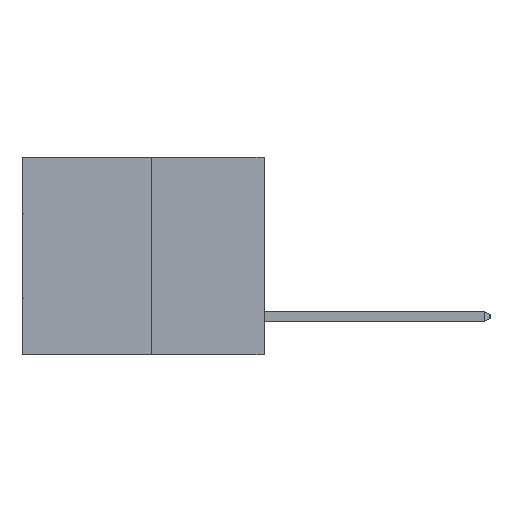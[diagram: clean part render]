
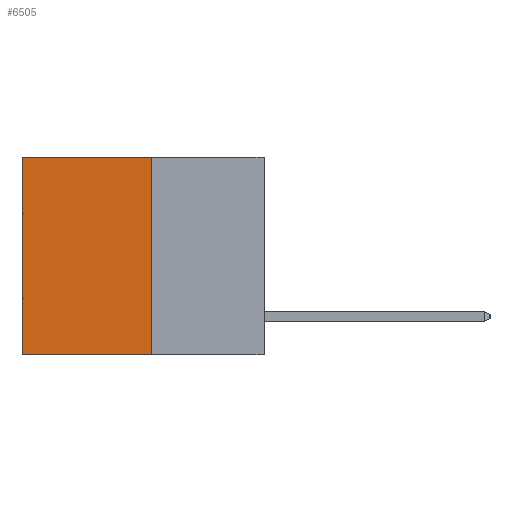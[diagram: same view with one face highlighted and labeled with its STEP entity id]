
A CAD part, left-side view. The second image highlights one B-rep face of the part: STEP entity #6505.
In plain terms, the highlighted planar face has unit normal (-1, 0, 0).
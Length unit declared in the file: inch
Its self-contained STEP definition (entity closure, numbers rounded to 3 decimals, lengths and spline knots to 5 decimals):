
#499 = FACE_OUTER_BOUND ( 'NONE', #31432, .T. ) ;
#2047 = EDGE_CURVE ( 'NONE', #15232, #29838, #20051, .T. ) ;
#3151 = LINE ( 'NONE', #14437, #3948 ) ;
#3948 = VECTOR ( 'NONE', #19595, 39.37008 ) ;
#3957 = VECTOR ( 'NONE', #15817, 39.37008 ) ;
#4215 = CARTESIAN_POINT ( 'NONE',  ( 0.3165, 0.6, 0. ) ) ;
#4527 = DIRECTION ( 'NONE',  ( 0., 0., -1. ) ) ;
#4625 = CARTESIAN_POINT ( 'NONE',  ( 0.3165, 0.28, 0. ) ) ;
#6505 = ADVANCED_FACE ( 'NONE', ( #499 ), #17336, .F. ) ;
#6701 = ORIENTED_EDGE ( 'NONE', *, *, #32404, .T. ) ;
#11124 = CARTESIAN_POINT ( 'NONE',  ( 0.3165, 0.6, -0.49 ) ) ;
#12651 = VERTEX_POINT ( 'NONE', #23319 ) ;
#14437 = CARTESIAN_POINT ( 'NONE',  ( 0.3165, 0.28, -0.49 ) ) ;
#15173 = EDGE_CURVE ( 'NONE', #12651, #21484, #23212, .T. ) ;
#15232 = VERTEX_POINT ( 'NONE', #22230 ) ;
#15817 = DIRECTION ( 'NONE',  ( 0., 0., -1. ) ) ;
#16692 = CARTESIAN_POINT ( 'NONE',  ( 0.3165, 0.28, -0.49 ) ) ;
#16719 = EDGE_CURVE ( 'NONE', #15232, #12651, #3151, .T. ) ;
#17330 = DIRECTION ( 'NONE',  ( 0., 1., 0. ) ) ;
#17336 = PLANE ( 'NONE',  #18341 ) ;
#17693 = VECTOR ( 'NONE', #17330, 39.37008 ) ;
#18341 = AXIS2_PLACEMENT_3D ( 'NONE', #19544, #24672, #4527 ) ;
#19544 = CARTESIAN_POINT ( 'NONE',  ( 0.3165, 0.28, -0.49 ) ) ;
#19595 = DIRECTION ( 'NONE',  ( 0., 0., -1. ) ) ;
#20051 = LINE ( 'NONE', #4625, #17693 ) ;
#20901 = CARTESIAN_POINT ( 'NONE',  ( 0.3165, 0.6, -0.49 ) ) ;
#21484 = VERTEX_POINT ( 'NONE', #20901 ) ;
#22230 = CARTESIAN_POINT ( 'NONE',  ( 0.3165, 0.28, 0. ) ) ;
#23212 = LINE ( 'NONE', #16692, #32240 ) ;
#23319 = CARTESIAN_POINT ( 'NONE',  ( 0.3165, 0.28, -0.49 ) ) ;
#23691 = ORIENTED_EDGE ( 'NONE', *, *, #16719, .F. ) ;
#24333 = DIRECTION ( 'NONE',  ( 0., 1., 0. ) ) ;
#24672 = DIRECTION ( 'NONE',  ( 1., 0., 0. ) ) ;
#25422 = ORIENTED_EDGE ( 'NONE', *, *, #15173, .F. ) ;
#29046 = LINE ( 'NONE', #11124, #3957 ) ;
#29838 = VERTEX_POINT ( 'NONE', #4215 ) ;
#30624 = ORIENTED_EDGE ( 'NONE', *, *, #2047, .T. ) ;
#31432 = EDGE_LOOP ( 'NONE', ( #6701, #25422, #23691, #30624 ) ) ;
#32240 = VECTOR ( 'NONE', #24333, 39.37008 ) ;
#32404 = EDGE_CURVE ( 'NONE', #29838, #21484, #29046, .T. ) ;
